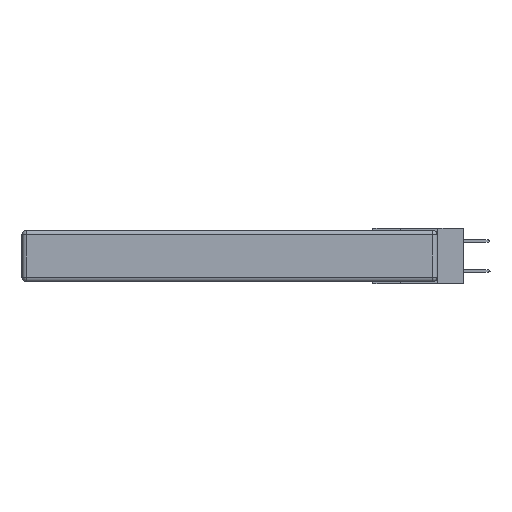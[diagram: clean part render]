
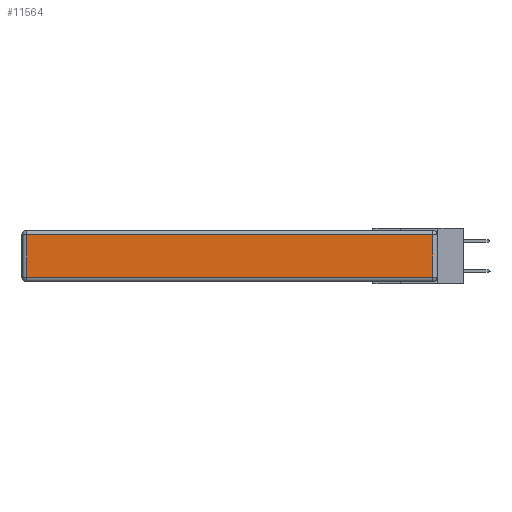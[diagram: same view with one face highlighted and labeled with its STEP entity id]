
A CAD part, left-side view. The second image highlights one B-rep face of the part: STEP entity #11564.
In plain terms, the highlighted planar face has unit normal (-1, 0, 0).
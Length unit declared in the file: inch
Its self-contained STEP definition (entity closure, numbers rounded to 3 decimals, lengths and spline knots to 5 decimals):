
#112 = ORIENTED_EDGE ( 'NONE', *, *, #18683, .T. ) ;
#141 = PLANE ( 'NONE',  #8900 ) ;
#588 = CARTESIAN_POINT ( 'NONE',  ( 0., 0.03, -0.343 ) ) ;
#1123 = VECTOR ( 'NONE', #17010, 39.37008 ) ;
#1164 = VECTOR ( 'NONE', #12459, 39.37008 ) ;
#1488 = EDGE_LOOP ( 'NONE', ( #21294, #2755, #112, #21168 ) ) ;
#1965 = CARTESIAN_POINT ( 'NONE',  ( 0., 2.72, -0.313 ) ) ;
#2213 = DIRECTION ( 'NONE',  ( -1., 0., 0. ) ) ;
#2338 = DIRECTION ( 'NONE',  ( 0., 0., 1. ) ) ;
#2523 = VECTOR ( 'NONE', #2338, 39.37008 ) ;
#2755 = ORIENTED_EDGE ( 'NONE', *, *, #3540, .T. ) ;
#3540 = EDGE_CURVE ( 'NONE', #12285, #7912, #7318, .T. ) ;
#4643 = EDGE_CURVE ( 'NONE', #11824, #5243, #9980, .T. ) ;
#5243 = VERTEX_POINT ( 'NONE', #1965 ) ;
#5464 = CARTESIAN_POINT ( 'NONE',  ( 0., 0.03, -0.313 ) ) ;
#6993 = VECTOR ( 'NONE', #20534, 39.37008 ) ;
#7318 = LINE ( 'NONE', #588, #2523 ) ;
#7912 = VERTEX_POINT ( 'NONE', #16787 ) ;
#8635 = CARTESIAN_POINT ( 'NONE',  ( 0., 2.75, -0.03 ) ) ;
#8900 = AXIS2_PLACEMENT_3D ( 'NONE', #17345, #2213, #20891 ) ;
#9980 = LINE ( 'NONE', #12922, #6993 ) ;
#11564 = ADVANCED_FACE ( 'NONE', ( #24339 ), #141, .T. ) ;
#11824 = VERTEX_POINT ( 'NONE', #16188 ) ;
#12285 = VERTEX_POINT ( 'NONE', #5464 ) ;
#12459 = DIRECTION ( 'NONE',  ( 0., 1., 0. ) ) ;
#12922 = CARTESIAN_POINT ( 'NONE',  ( 0., 2.72, -0.343 ) ) ;
#16188 = CARTESIAN_POINT ( 'NONE',  ( 0., 2.72, -0.03 ) ) ;
#16787 = CARTESIAN_POINT ( 'NONE',  ( 0., 0.03, -0.03 ) ) ;
#17010 = DIRECTION ( 'NONE',  ( 0., -1., 0. ) ) ;
#17345 = CARTESIAN_POINT ( 'NONE',  ( 0., 0., -0.343 ) ) ;
#18669 = CARTESIAN_POINT ( 'NONE',  ( 0., 0., -0.313 ) ) ;
#18683 = EDGE_CURVE ( 'NONE', #7912, #11824, #20194, .T. ) ;
#19340 = EDGE_CURVE ( 'NONE', #5243, #12285, #20155, .T. ) ;
#20155 = LINE ( 'NONE', #18669, #1123 ) ;
#20194 = LINE ( 'NONE', #8635, #1164 ) ;
#20534 = DIRECTION ( 'NONE',  ( 0., 0., -1. ) ) ;
#20891 = DIRECTION ( 'NONE',  ( 0., 0., 1. ) ) ;
#21168 = ORIENTED_EDGE ( 'NONE', *, *, #4643, .T. ) ;
#21294 = ORIENTED_EDGE ( 'NONE', *, *, #19340, .T. ) ;
#24339 = FACE_OUTER_BOUND ( 'NONE', #1488, .T. ) ;
